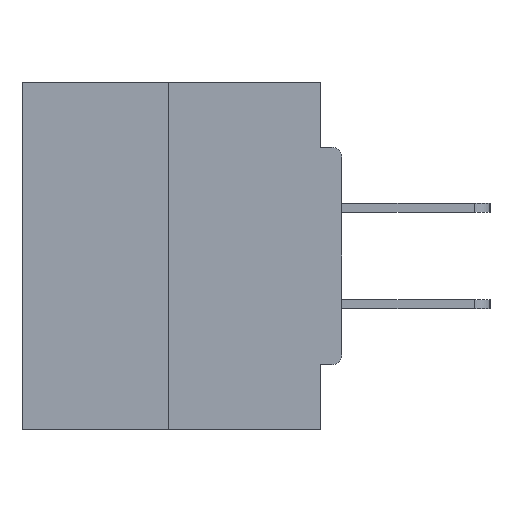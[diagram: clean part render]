
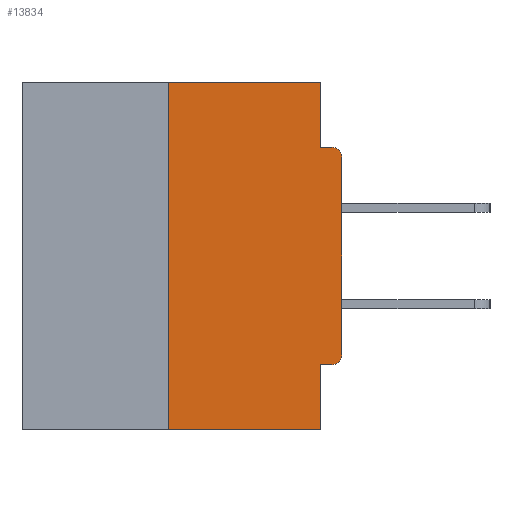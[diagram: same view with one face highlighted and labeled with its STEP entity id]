
A CAD part, left-side view. The second image highlights one B-rep face of the part: STEP entity #13834.
In plain terms, the highlighted planar face has unit normal (-1, 0, 0).
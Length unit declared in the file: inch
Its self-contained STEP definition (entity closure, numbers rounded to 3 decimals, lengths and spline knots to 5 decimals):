
#254 = EDGE_CURVE ( 'NONE', #18159, #29408, #18700, .T. ) ;
#883 = CARTESIAN_POINT ( 'NONE',  ( 0., 0., -0.3915 ) ) ;
#2808 = CARTESIAN_POINT ( 'NONE',  ( 0., 0., -0.1085 ) ) ;
#2951 = DIRECTION ( 'NONE',  ( 0., -1., 0. ) ) ;
#3109 = CARTESIAN_POINT ( 'NONE',  ( 0., 0.46, -0.5 ) ) ;
#4413 = VECTOR ( 'NONE', #8709, 39.37008 ) ;
#4530 = VECTOR ( 'NONE', #11580, 39.37008 ) ;
#4593 = CARTESIAN_POINT ( 'NONE',  ( 0., 0.031, -0.4065 ) ) ;
#4647 = ORIENTED_EDGE ( 'NONE', *, *, #15437, .F. ) ;
#4764 = EDGE_CURVE ( 'NONE', #32731, #23495, #5218, .T. ) ;
#5218 = CIRCLE ( 'NONE', #7142, 0.015 ) ;
#5641 = CARTESIAN_POINT ( 'NONE',  ( 0., 0., -0.4065 ) ) ;
#6564 = CARTESIAN_POINT ( 'NONE',  ( 0., 0.031, 0. ) ) ;
#7082 = CARTESIAN_POINT ( 'NONE',  ( 0., 0.031, -0.0935 ) ) ;
#7142 = AXIS2_PLACEMENT_3D ( 'NONE', #7693, #13690, #25665 ) ;
#7693 = CARTESIAN_POINT ( 'NONE',  ( 0., 0.015, -0.1085 ) ) ;
#8088 = DIRECTION ( 'NONE',  ( 0., 0., 1. ) ) ;
#8283 = VERTEX_POINT ( 'NONE', #34339 ) ;
#8550 = LINE ( 'NONE', #31630, #4413 ) ;
#8709 = DIRECTION ( 'NONE',  ( 0., 0., 1. ) ) ;
#9017 = EDGE_CURVE ( 'NONE', #26801, #32731, #15142, .T. ) ;
#9607 = EDGE_CURVE ( 'NONE', #19516, #29408, #12302, .T. ) ;
#10917 = VECTOR ( 'NONE', #37879, 39.37008 ) ;
#11099 = FACE_OUTER_BOUND ( 'NONE', #32715, .T. ) ;
#11485 = CARTESIAN_POINT ( 'NONE',  ( 0., 0.031, 0. ) ) ;
#11580 = DIRECTION ( 'NONE',  ( 0., 0., -1. ) ) ;
#12299 = CARTESIAN_POINT ( 'NONE',  ( 0., 0.015, -0.0935 ) ) ;
#12302 = LINE ( 'NONE', #20751, #4530 ) ;
#12477 = EDGE_CURVE ( 'NONE', #36102, #26801, #30778, .T. ) ;
#12680 = VECTOR ( 'NONE', #35589, 39.37008 ) ;
#13690 = DIRECTION ( 'NONE',  ( -1., 0., 0. ) ) ;
#13834 = ADVANCED_FACE ( 'NONE', ( #11099 ), #21805, .F. ) ;
#14336 = ORIENTED_EDGE ( 'NONE', *, *, #9607, .F. ) ;
#14349 = ORIENTED_EDGE ( 'NONE', *, *, #37360, .F. ) ;
#14411 = CARTESIAN_POINT ( 'NONE',  ( 0., 0.25, -0.5 ) ) ;
#14673 = DIRECTION ( 'NONE',  ( -1., 0., 0. ) ) ;
#15059 = CARTESIAN_POINT ( 'NONE',  ( 0., 0.015, -0.4065 ) ) ;
#15142 = LINE ( 'NONE', #34658, #18345 ) ;
#15437 = EDGE_CURVE ( 'NONE', #8283, #19071, #33010, .T. ) ;
#16161 = ORIENTED_EDGE ( 'NONE', *, *, #9017, .T. ) ;
#16216 = DIRECTION ( 'NONE',  ( 0., -1., 0. ) ) ;
#16362 = VECTOR ( 'NONE', #20562, 39.37008 ) ;
#17473 = ORIENTED_EDGE ( 'NONE', *, *, #4764, .T. ) ;
#18159 = VERTEX_POINT ( 'NONE', #14411 ) ;
#18345 = VECTOR ( 'NONE', #8088, 39.37008 ) ;
#18700 = LINE ( 'NONE', #3109, #10917 ) ;
#19036 = CARTESIAN_POINT ( 'NONE',  ( 0., 0.46, 0. ) ) ;
#19071 = VERTEX_POINT ( 'NONE', #6564 ) ;
#19152 = DIRECTION ( 'NONE',  ( 1., 0., 0. ) ) ;
#19516 = VERTEX_POINT ( 'NONE', #4593 ) ;
#20562 = DIRECTION ( 'NONE',  ( 0., 1., 0. ) ) ;
#20642 = LINE ( 'NONE', #32054, #24701 ) ;
#20751 = CARTESIAN_POINT ( 'NONE',  ( 0., 0.031, -0.5 ) ) ;
#21805 = PLANE ( 'NONE',  #36706 ) ;
#21914 = EDGE_CURVE ( 'NONE', #19071, #35548, #28678, .T. ) ;
#23495 = VERTEX_POINT ( 'NONE', #12299 ) ;
#24072 = ORIENTED_EDGE ( 'NONE', *, *, #30823, .F. ) ;
#24701 = VECTOR ( 'NONE', #2951, 39.37008 ) ;
#24716 = DIRECTION ( 'NONE',  ( 0., 0., -1. ) ) ;
#25665 = DIRECTION ( 'NONE',  ( 0., 0., -1. ) ) ;
#26330 = ORIENTED_EDGE ( 'NONE', *, *, #254, .T. ) ;
#26801 = VERTEX_POINT ( 'NONE', #883 ) ;
#27531 = VECTOR ( 'NONE', #16216, 39.37008 ) ;
#27913 = CARTESIAN_POINT ( 'NONE',  ( 0., 0.46, 0. ) ) ;
#28053 = ORIENTED_EDGE ( 'NONE', *, *, #21914, .F. ) ;
#28678 = LINE ( 'NONE', #11485, #12680 ) ;
#29408 = VERTEX_POINT ( 'NONE', #35620 ) ;
#29437 = DIRECTION ( 'NONE',  ( 0., 0., -1. ) ) ;
#30778 = CIRCLE ( 'NONE', #33748, 0.015 ) ;
#30823 = EDGE_CURVE ( 'NONE', #35548, #23495, #20642, .T. ) ;
#31630 = CARTESIAN_POINT ( 'NONE',  ( 0., 0.25, 0. ) ) ;
#32007 = CARTESIAN_POINT ( 'NONE',  ( 0., 0.015, -0.3915 ) ) ;
#32054 = CARTESIAN_POINT ( 'NONE',  ( 0., 0., -0.0935 ) ) ;
#32715 = EDGE_LOOP ( 'NONE', ( #4647, #37332, #26330, #14336, #14349, #34137, #16161, #17473, #24072, #28053 ) ) ;
#32731 = VERTEX_POINT ( 'NONE', #2808 ) ;
#32782 = LINE ( 'NONE', #5641, #16362 ) ;
#33010 = LINE ( 'NONE', #19036, #27531 ) ;
#33360 = EDGE_CURVE ( 'NONE', #18159, #8283, #8550, .T. ) ;
#33748 = AXIS2_PLACEMENT_3D ( 'NONE', #32007, #14673, #29437 ) ;
#34137 = ORIENTED_EDGE ( 'NONE', *, *, #12477, .T. ) ;
#34339 = CARTESIAN_POINT ( 'NONE',  ( 0., 0.25, 0. ) ) ;
#34658 = CARTESIAN_POINT ( 'NONE',  ( 0., 0., 0. ) ) ;
#35548 = VERTEX_POINT ( 'NONE', #7082 ) ;
#35589 = DIRECTION ( 'NONE',  ( 0., 0., -1. ) ) ;
#35620 = CARTESIAN_POINT ( 'NONE',  ( 0., 0.031, -0.5 ) ) ;
#36102 = VERTEX_POINT ( 'NONE', #15059 ) ;
#36706 = AXIS2_PLACEMENT_3D ( 'NONE', #27913, #19152, #24716 ) ;
#37332 = ORIENTED_EDGE ( 'NONE', *, *, #33360, .F. ) ;
#37360 = EDGE_CURVE ( 'NONE', #36102, #19516, #32782, .T. ) ;
#37879 = DIRECTION ( 'NONE',  ( 0., -1., 0. ) ) ;
